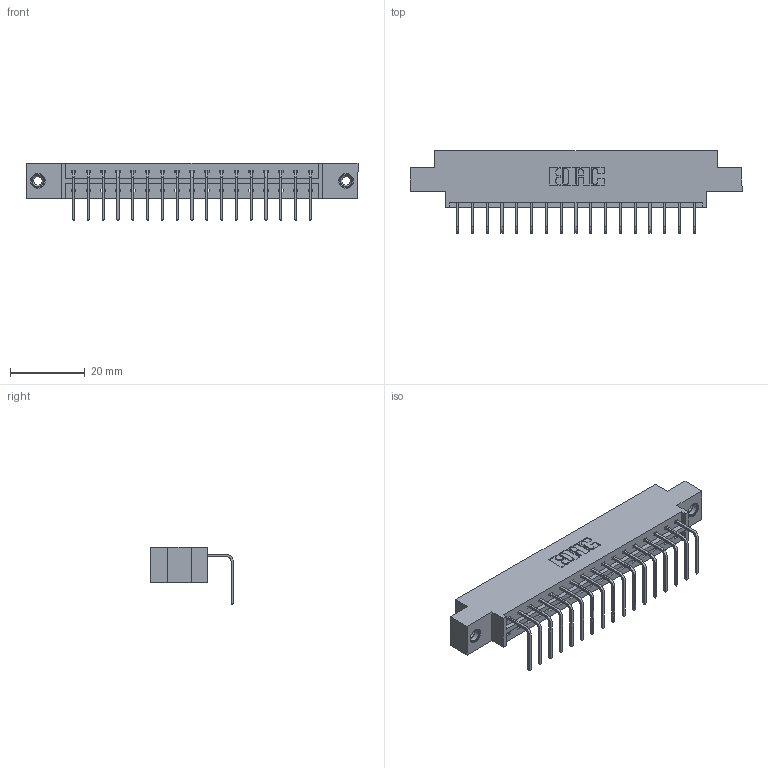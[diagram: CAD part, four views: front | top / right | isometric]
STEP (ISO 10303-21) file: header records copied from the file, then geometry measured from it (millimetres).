
FILE_DESCRIPTION (( 'STEP AP203' ), '1' );
FILE_NAME ('833-017-558-608.STEP', '2020-05-31T20:34:30', ( '' ), ( '' ), 'SwSTEP 2.0', 'SolidWorks 2020', '' );
FILE_SCHEMA (( 'CONFIG_CONTROL_DESIGN' ));
Length unit declared in the file: inch
Products named in the file (4): 833 Part_Offset - .156 Dia - TI; 345-250-001_345-250-003-102; 345-292-001_558 Tail - 2; 833-017-558-608
Assembly tree (20 placements, depth 2):
  833-017-558-608
    833 Part_Offset - .156 Dia - TI
    345-292-001_558 Tail - 2  x17
    345-250-001_345-250-003-102  x2
Bounding box: 88.9 x 22.17 x 15.37 mm (x, y, z)
Volume: 8553.2 mm3; surface area: 9661.9 mm2
Topology: 20 solids, 20 shells, 1198 faces, 3553 edges, 2338 vertices
Faces by surface type: plane 854, cylinder 328, cone 12, torus 4
Entity records: 15028 total; most frequent: CARTESIAN_POINT 2580, ORIENTED_EDGE 2526, DIRECTION 2259, EDGE_CURVE 1263, VECTOR 1115, LINE 1115, VERTEX_POINT 836, AXIS2_PLACEMENT_3D 572
